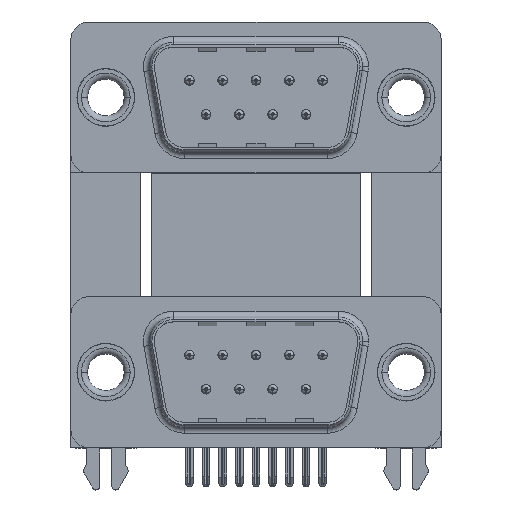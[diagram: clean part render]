
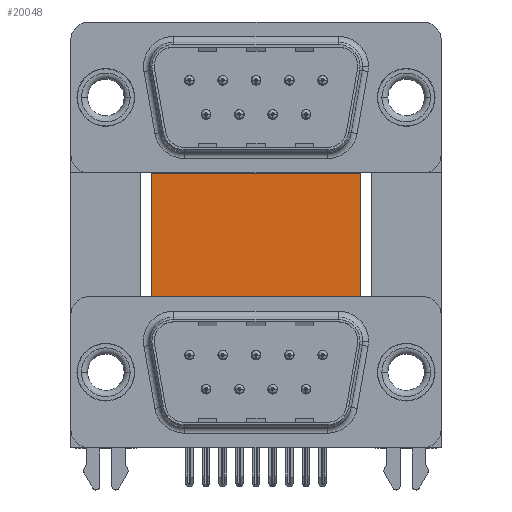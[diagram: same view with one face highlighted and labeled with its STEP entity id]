
A CAD part, top view. The second image highlights one B-rep face of the part: STEP entity #20048.
In plain terms, the highlighted planar face has unit normal (0, 0, 1).
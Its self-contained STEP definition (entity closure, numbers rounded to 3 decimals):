
#290 = VERTEX_POINT ( 'NONE', #19023 ) ;
#602 = VERTEX_POINT ( 'NONE', #13009 ) ;
#743 = CARTESIAN_POINT ( 'NONE',  ( 3.79, 16.585, -12. ) ) ;
#924 = DIRECTION ( 'NONE',  ( 1., 0., 0. ) ) ;
#1134 = DIRECTION ( 'NONE',  ( 1., 0., 0. ) ) ;
#1334 = VECTOR ( 'NONE', #2704, 1000. ) ;
#1603 = VECTOR ( 'NONE', #20921, 1000. ) ;
#2033 = VECTOR ( 'NONE', #924, 1000. ) ;
#2070 = CARTESIAN_POINT ( 'NONE',  ( 3.79, 16.585, -12. ) ) ;
#2116 = LINE ( 'NONE', #23791, #17098 ) ;
#2210 = ORIENTED_EDGE ( 'NONE', *, *, #10087, .F. ) ;
#2291 = VERTEX_POINT ( 'NONE', #12552 ) ;
#2427 = EDGE_CURVE ( 'NONE', #290, #13508, #14218, .T. ) ;
#2704 = DIRECTION ( 'NONE',  ( 1., 0., 0. ) ) ;
#3601 = DIRECTION ( 'NONE',  ( 0., -1., 0. ) ) ;
#3824 = LINE ( 'NONE', #7655, #1603 ) ;
#4117 = DIRECTION ( 'NONE',  ( -1., 0., 0. ) ) ;
#4533 = CARTESIAN_POINT ( 'NONE',  ( 2.4, -4.635, -12. ) ) ;
#4633 = VECTOR ( 'NONE', #3601, 1000. ) ;
#4896 = ORIENTED_EDGE ( 'NONE', *, *, #23108, .T. ) ;
#5799 = CARTESIAN_POINT ( 'NONE',  ( 21.2, -0.735, -12. ) ) ;
#6136 = VECTOR ( 'NONE', #24369, 1000. ) ;
#7655 = CARTESIAN_POINT ( 'NONE',  ( 2.9, -4.635, -12. ) ) ;
#7754 = LINE ( 'NONE', #15526, #21157 ) ;
#8805 = LINE ( 'NONE', #18236, #25196 ) ;
#9844 = DIRECTION ( 'NONE',  ( 0., 0., -1. ) ) ;
#10087 = EDGE_CURVE ( 'NONE', #2291, #11392, #24613, .T. ) ;
#10162 = ORIENTED_EDGE ( 'NONE', *, *, #2427, .T. ) ;
#10261 = ORIENTED_EDGE ( 'NONE', *, *, #22687, .T. ) ;
#10470 = CARTESIAN_POINT ( 'NONE',  ( 22.09, -4.635, -12. ) ) ;
#11392 = VERTEX_POINT ( 'NONE', #17762 ) ;
#11660 = VECTOR ( 'NONE', #1134, 1000. ) ;
#11814 = DIRECTION ( 'NONE',  ( -0.336, 0.942, 0. ) ) ;
#11887 = CARTESIAN_POINT ( 'NONE',  ( 22.59, -4.635, -12. ) ) ;
#11937 = EDGE_CURVE ( 'NONE', #602, #15516, #8805, .T. ) ;
#12098 = CARTESIAN_POINT ( 'NONE',  ( 2.4, -4.635, -12. ) ) ;
#12177 = DIRECTION ( 'NONE',  ( 0., -1., 0. ) ) ;
#12217 = CARTESIAN_POINT ( 'NONE',  ( 22.09, -3.735, -12. ) ) ;
#12512 = ORIENTED_EDGE ( 'NONE', *, *, #11937, .T. ) ;
#12552 = CARTESIAN_POINT ( 'NONE',  ( 3.79, 16.585, -12. ) ) ;
#12919 = ORIENTED_EDGE ( 'NONE', *, *, #22187, .F. ) ;
#13009 = CARTESIAN_POINT ( 'NONE',  ( 2.9, -4.635, -12. ) ) ;
#13508 = VERTEX_POINT ( 'NONE', #12098 ) ;
#13543 = CARTESIAN_POINT ( 'NONE',  ( 21.2, 16.585, -12. ) ) ;
#14218 = LINE ( 'NONE', #4533, #16929 ) ;
#14259 = EDGE_CURVE ( 'NONE', #20000, #14664, #7754, .T. ) ;
#14266 = ORIENTED_EDGE ( 'NONE', *, *, #15360, .T. ) ;
#14477 = ORIENTED_EDGE ( 'NONE', *, *, #14829, .T. ) ;
#14582 = CARTESIAN_POINT ( 'NONE',  ( 3.79, -3.735, -12. ) ) ;
#14664 = VERTEX_POINT ( 'NONE', #5799 ) ;
#14829 = EDGE_CURVE ( 'NONE', #15516, #24078, #20709, .T. ) ;
#15360 = EDGE_CURVE ( 'NONE', #24078, #16540, #16585, .T. ) ;
#15516 = VERTEX_POINT ( 'NONE', #21057 ) ;
#15526 = CARTESIAN_POINT ( 'NONE',  ( 22.59, -4.635, -12. ) ) ;
#16540 = VERTEX_POINT ( 'NONE', #10470 ) ;
#16585 = LINE ( 'NONE', #22592, #6136 ) ;
#16929 = VECTOR ( 'NONE', #20082, 1000. ) ;
#17098 = VECTOR ( 'NONE', #12177, 1000. ) ;
#17762 = CARTESIAN_POINT ( 'NONE',  ( 21.2, 16.585, -12. ) ) ;
#18126 = LINE ( 'NONE', #20434, #1334 ) ;
#18236 = CARTESIAN_POINT ( 'NONE',  ( 2.9, -3.735, -12. ) ) ;
#18759 = DIRECTION ( 'NONE',  ( 0., 1., 0. ) ) ;
#19023 = CARTESIAN_POINT ( 'NONE',  ( 3.79, -0.735, -12. ) ) ;
#20000 = VERTEX_POINT ( 'NONE', #11887 ) ;
#20048 = ADVANCED_FACE ( 'NONE', ( #21589 ), #23373, .F. ) ;
#20082 = DIRECTION ( 'NONE',  ( -0.336, -0.942, 0. ) ) ;
#20112 = ORIENTED_EDGE ( 'NONE', *, *, #21471, .T. ) ;
#20434 = CARTESIAN_POINT ( 'NONE',  ( 22.09, -4.635, -12. ) ) ;
#20709 = LINE ( 'NONE', #14582, #2033 ) ;
#20921 = DIRECTION ( 'NONE',  ( 1., 0., 0. ) ) ;
#20929 = ORIENTED_EDGE ( 'NONE', *, *, #14259, .T. ) ;
#20953 = LINE ( 'NONE', #13543, #4633 ) ;
#21057 = CARTESIAN_POINT ( 'NONE',  ( 2.9, -3.735, -12. ) ) ;
#21157 = VECTOR ( 'NONE', #11814, 1000. ) ;
#21471 = EDGE_CURVE ( 'NONE', #16540, #20000, #18126, .T. ) ;
#21589 = FACE_OUTER_BOUND ( 'NONE', #21850, .T. ) ;
#21850 = EDGE_LOOP ( 'NONE', ( #14477, #14266, #20112, #20929, #12919, #2210, #4896, #10162, #10261, #12512 ) ) ;
#22187 = EDGE_CURVE ( 'NONE', #11392, #14664, #20953, .T. ) ;
#22592 = CARTESIAN_POINT ( 'NONE',  ( 22.09, -3.735, -12. ) ) ;
#22687 = EDGE_CURVE ( 'NONE', #13508, #602, #3824, .T. ) ;
#23108 = EDGE_CURVE ( 'NONE', #2291, #290, #2116, .T. ) ;
#23289 = AXIS2_PLACEMENT_3D ( 'NONE', #2070, #9844, #4117 ) ;
#23373 = PLANE ( 'NONE',  #23289 ) ;
#23791 = CARTESIAN_POINT ( 'NONE',  ( 3.79, 16.585, -12. ) ) ;
#24078 = VERTEX_POINT ( 'NONE', #12217 ) ;
#24369 = DIRECTION ( 'NONE',  ( 0., -1., 0. ) ) ;
#24613 = LINE ( 'NONE', #743, #11660 ) ;
#25196 = VECTOR ( 'NONE', #18759, 1000. ) ;
